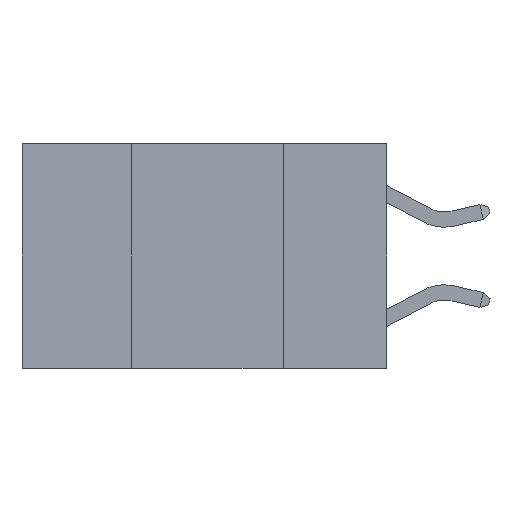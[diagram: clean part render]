
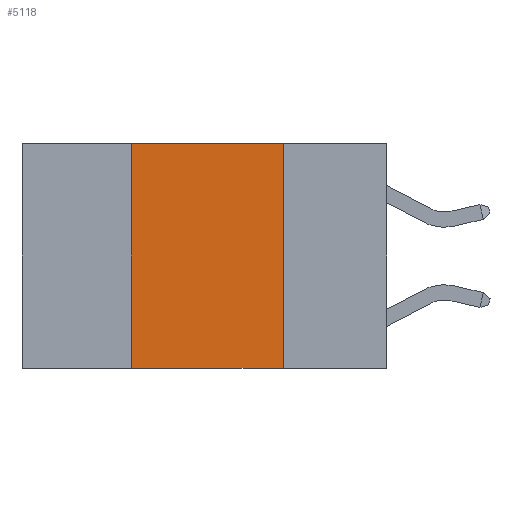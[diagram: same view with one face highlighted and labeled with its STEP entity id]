
A CAD part, left-side view. The second image highlights one B-rep face of the part: STEP entity #5118.
In plain terms, the highlighted planar face has unit normal (-1, 0, 0).
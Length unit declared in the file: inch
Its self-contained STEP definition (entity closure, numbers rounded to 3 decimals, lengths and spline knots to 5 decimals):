
#262 = FACE_OUTER_BOUND ( 'NONE', #3961, .T. ) ;
#311 = ORIENTED_EDGE ( 'NONE', *, *, #3646, .F. ) ;
#1197 = LINE ( 'NONE', #6797, #6218 ) ;
#1832 = VERTEX_POINT ( 'NONE', #5325 ) ;
#1887 = EDGE_CURVE ( 'NONE', #2094, #6177, #2694, .T. ) ;
#1932 = LINE ( 'NONE', #8910, #7170 ) ;
#2094 = VERTEX_POINT ( 'NONE', #5716 ) ;
#2254 = VECTOR ( 'NONE', #3065, 39.37008 ) ;
#2694 = LINE ( 'NONE', #5362, #6126 ) ;
#2701 = VERTEX_POINT ( 'NONE', #8164 ) ;
#2894 = LINE ( 'NONE', #6444, #2254 ) ;
#3065 = DIRECTION ( 'NONE',  ( 0., -1., 0. ) ) ;
#3117 = EDGE_CURVE ( 'NONE', #1832, #2701, #2894, .T. ) ;
#3490 = ORIENTED_EDGE ( 'NONE', *, *, #1887, .F. ) ;
#3548 = EDGE_CURVE ( 'NONE', #1832, #2094, #1197, .T. ) ;
#3646 = EDGE_CURVE ( 'NONE', #6177, #2701, #1932, .T. ) ;
#3830 = AXIS2_PLACEMENT_3D ( 'NONE', #5999, #8680, #4627 ) ;
#3961 = EDGE_LOOP ( 'NONE', ( #311, #3490, #8389, #5992 ) ) ;
#4085 = DIRECTION ( 'NONE',  ( 0., 0., 1. ) ) ;
#4627 = DIRECTION ( 'NONE',  ( 0., 0., -1. ) ) ;
#4874 = DIRECTION ( 'NONE',  ( 0., 0., -1. ) ) ;
#5118 = ADVANCED_FACE ( 'NONE', ( #262 ), #8031, .F. ) ;
#5325 = CARTESIAN_POINT ( 'NONE',  ( 0., 0.42, -0.37 ) ) ;
#5362 = CARTESIAN_POINT ( 'NONE',  ( 0., 0.6, 0. ) ) ;
#5716 = CARTESIAN_POINT ( 'NONE',  ( 0., 0.42, 0. ) ) ;
#5992 = ORIENTED_EDGE ( 'NONE', *, *, #3117, .T. ) ;
#5999 = CARTESIAN_POINT ( 'NONE',  ( 0., 0.6, 0. ) ) ;
#6126 = VECTOR ( 'NONE', #6722, 39.37008 ) ;
#6177 = VERTEX_POINT ( 'NONE', #6686 ) ;
#6218 = VECTOR ( 'NONE', #4085, 39.37008 ) ;
#6444 = CARTESIAN_POINT ( 'NONE',  ( 0., 0.6, -0.37 ) ) ;
#6686 = CARTESIAN_POINT ( 'NONE',  ( 0., 0.17, 0. ) ) ;
#6722 = DIRECTION ( 'NONE',  ( 0., -1., 0. ) ) ;
#6797 = CARTESIAN_POINT ( 'NONE',  ( 0., 0.42, 0. ) ) ;
#7170 = VECTOR ( 'NONE', #4874, 39.37008 ) ;
#8031 = PLANE ( 'NONE',  #3830 ) ;
#8164 = CARTESIAN_POINT ( 'NONE',  ( 0., 0.17, -0.37 ) ) ;
#8389 = ORIENTED_EDGE ( 'NONE', *, *, #3548, .F. ) ;
#8680 = DIRECTION ( 'NONE',  ( 1., 0., 0. ) ) ;
#8910 = CARTESIAN_POINT ( 'NONE',  ( 0., 0.17, 0. ) ) ;
